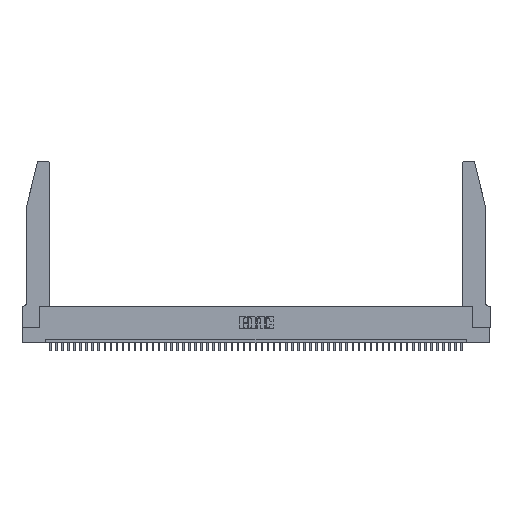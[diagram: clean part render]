
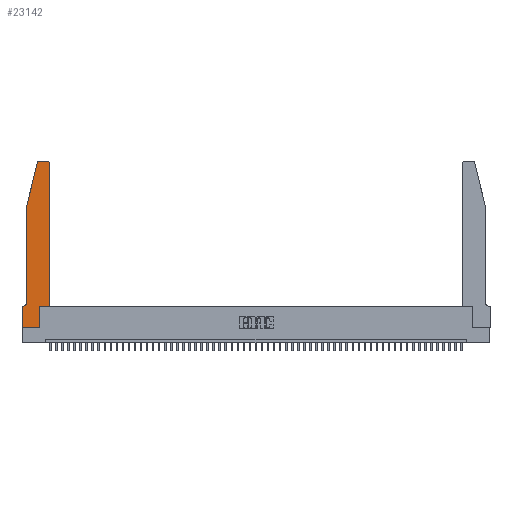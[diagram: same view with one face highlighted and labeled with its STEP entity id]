
A CAD part, top view. The second image highlights one B-rep face of the part: STEP entity #23142.
In plain terms, the highlighted planar face has unit normal (0, 0, 1).
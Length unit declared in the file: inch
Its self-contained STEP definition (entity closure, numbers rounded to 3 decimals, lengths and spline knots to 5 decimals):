
#243 = EDGE_LOOP ( 'NONE', ( #18158, #18048, #43038, #37399, #42658, #34288, #34234, #25172, #28379, #49204, #23514, #32683 ) ) ;
#1354 = LINE ( 'NONE', #51757, #47501 ) ;
#1744 = DIRECTION ( 'NONE',  ( 1., 0., 0. ) ) ;
#2928 = AXIS2_PLACEMENT_3D ( 'NONE', #8371, #4436, #11940 ) ;
#3563 = DIRECTION ( 'NONE',  ( -0.239, -0.971, 0. ) ) ;
#4314 = VERTEX_POINT ( 'NONE', #22705 ) ;
#4436 = DIRECTION ( 'NONE',  ( 0., 0., 1. ) ) ;
#4733 = VERTEX_POINT ( 'NONE', #39611 ) ;
#5491 = CARTESIAN_POINT ( 'NONE',  ( 0.4205, 2.72, 0.37 ) ) ;
#6585 = DIRECTION ( 'NONE',  ( 0., -1., 0. ) ) ;
#7000 = EDGE_CURVE ( 'NONE', #42185, #9568, #35794, .T. ) ;
#7491 = CARTESIAN_POINT ( 'NONE',  ( 0.0755, 2., 0.37 ) ) ;
#8063 = DIRECTION ( 'NONE',  ( 0., -1., 0. ) ) ;
#8371 = CARTESIAN_POINT ( 'NONE',  ( 0.284, 2.72, 0.37 ) ) ;
#9288 = LINE ( 'NONE', #7491, #38144 ) ;
#9568 = VERTEX_POINT ( 'NONE', #14014 ) ;
#9901 = LINE ( 'NONE', #24311, #46450 ) ;
#11267 = VECTOR ( 'NONE', #15106, 39.37008 ) ;
#11940 = DIRECTION ( 'NONE',  ( 1., 0., 0. ) ) ;
#13258 = VERTEX_POINT ( 'NONE', #42919 ) ;
#14014 = CARTESIAN_POINT ( 'NONE',  ( 0., 0.35, 0.37 ) ) ;
#14015 = VERTEX_POINT ( 'NONE', #36875 ) ;
#14400 = EDGE_CURVE ( 'NONE', #44410, #52552, #49768, .T. ) ;
#14858 = AXIS2_PLACEMENT_3D ( 'NONE', #26701, #46902, #34383 ) ;
#15106 = DIRECTION ( 'NONE',  ( -1., 0., 0. ) ) ;
#15272 = VECTOR ( 'NONE', #31487, 39.37008 ) ;
#18048 = ORIENTED_EDGE ( 'NONE', *, *, #46040, .T. ) ;
#18158 = ORIENTED_EDGE ( 'NONE', *, *, #37678, .T. ) ;
#18743 = DIRECTION ( 'NONE',  ( 1., 0., 0. ) ) ;
#19446 = CARTESIAN_POINT ( 'NONE',  ( 0.0755, 0.35, 0.37 ) ) ;
#20597 = CARTESIAN_POINT ( 'NONE',  ( 0.0055, 0.35, 0.37 ) ) ;
#20752 = CIRCLE ( 'NONE', #14858, 0.07 ) ;
#22087 = DIRECTION ( 'NONE',  ( 1., 0., 0. ) ) ;
#22111 = EDGE_CURVE ( 'NONE', #49598, #33706, #38552, .T. ) ;
#22705 = CARTESIAN_POINT ( 'NONE',  ( 0., 0., 0.37 ) ) ;
#23142 = ADVANCED_FACE ( 'NONE', ( #51906 ), #30871, .T. ) ;
#23167 = DIRECTION ( 'NONE',  ( 0., 0., 1. ) ) ;
#23514 = ORIENTED_EDGE ( 'NONE', *, *, #40303, .T. ) ;
#24285 = EDGE_CURVE ( 'NONE', #4314, #13258, #43099, .T. ) ;
#24311 = CARTESIAN_POINT ( 'NONE',  ( 0.2865, 0.35, 0.37 ) ) ;
#25172 = ORIENTED_EDGE ( 'NONE', *, *, #24285, .T. ) ;
#26701 = CARTESIAN_POINT ( 'NONE',  ( 0.0055, 0.42, 0.37 ) ) ;
#27271 = DIRECTION ( 'NONE',  ( 1., 0., 0. ) ) ;
#27760 = CARTESIAN_POINT ( 'NONE',  ( 0.4505, 2.72, 0.37 ) ) ;
#28379 = ORIENTED_EDGE ( 'NONE', *, *, #53070, .T. ) ;
#28793 = LINE ( 'NONE', #34871, #29410 ) ;
#29410 = VECTOR ( 'NONE', #51356, 39.37008 ) ;
#30864 = EDGE_CURVE ( 'NONE', #9568, #4314, #1354, .T. ) ;
#30871 = PLANE ( 'NONE',  #45918 ) ;
#31487 = DIRECTION ( 'NONE',  ( -1., 0., 0. ) ) ;
#32683 = ORIENTED_EDGE ( 'NONE', *, *, #14400, .T. ) ;
#32839 = CARTESIAN_POINT ( 'NONE',  ( 0.0755, 2., 0.37 ) ) ;
#32905 = VECTOR ( 'NONE', #18743, 39.37008 ) ;
#33039 = EDGE_CURVE ( 'NONE', #4733, #42185, #20752, .T. ) ;
#33077 = DIRECTION ( 'NONE',  ( 0., 1., 0. ) ) ;
#33706 = VERTEX_POINT ( 'NONE', #46467 ) ;
#34234 = ORIENTED_EDGE ( 'NONE', *, *, #30864, .T. ) ;
#34288 = ORIENTED_EDGE ( 'NONE', *, *, #7000, .T. ) ;
#34333 = CARTESIAN_POINT ( 'NONE',  ( 0., 0., 0.37 ) ) ;
#34354 = CIRCLE ( 'NONE', #2928, 0.03 ) ;
#34383 = DIRECTION ( 'NONE',  ( -1., 0., 0. ) ) ;
#34656 = CARTESIAN_POINT ( 'NONE',  ( 0.25487, 2.72718, 0.37 ) ) ;
#34871 = CARTESIAN_POINT ( 'NONE',  ( 0.4505, 0.35, 0.37 ) ) ;
#35746 = AXIS2_PLACEMENT_3D ( 'NONE', #5491, #50836, #1744 ) ;
#35794 = LINE ( 'NONE', #19446, #15272 ) ;
#36589 = VECTOR ( 'NONE', #8063, 39.37008 ) ;
#36875 = CARTESIAN_POINT ( 'NONE',  ( 0.284, 2.75, 0.37 ) ) ;
#37399 = ORIENTED_EDGE ( 'NONE', *, *, #39576, .T. ) ;
#37678 = EDGE_CURVE ( 'NONE', #52552, #14015, #42075, .T. ) ;
#37771 = VERTEX_POINT ( 'NONE', #53056 ) ;
#38144 = VECTOR ( 'NONE', #3563, 39.37008 ) ;
#38442 = EDGE_CURVE ( 'NONE', #39146, #37771, #9288, .T. ) ;
#38552 = LINE ( 'NONE', #38573, #42374 ) ;
#38573 = CARTESIAN_POINT ( 'NONE',  ( 0.4505, 0.35, 0.37 ) ) ;
#39146 = VERTEX_POINT ( 'NONE', #34656 ) ;
#39576 = EDGE_CURVE ( 'NONE', #37771, #4733, #49403, .T. ) ;
#39593 = CARTESIAN_POINT ( 'NONE',  ( 0., 0.35, 0.37 ) ) ;
#39611 = CARTESIAN_POINT ( 'NONE',  ( 0.0755, 0.42, 0.37 ) ) ;
#40303 = EDGE_CURVE ( 'NONE', #33706, #44410, #28793, .T. ) ;
#42075 = LINE ( 'NONE', #47883, #11267 ) ;
#42185 = VERTEX_POINT ( 'NONE', #20597 ) ;
#42374 = VECTOR ( 'NONE', #22087, 39.37008 ) ;
#42658 = ORIENTED_EDGE ( 'NONE', *, *, #33039, .T. ) ;
#42919 = CARTESIAN_POINT ( 'NONE',  ( 0.2865, 0., 0.37 ) ) ;
#43038 = ORIENTED_EDGE ( 'NONE', *, *, #38442, .T. ) ;
#43099 = LINE ( 'NONE', #34333, #32905 ) ;
#44410 = VERTEX_POINT ( 'NONE', #27760 ) ;
#45429 = CARTESIAN_POINT ( 'NONE',  ( 0.4205, 2.75, 0.37 ) ) ;
#45918 = AXIS2_PLACEMENT_3D ( 'NONE', #39593, #23167, #27271 ) ;
#46040 = EDGE_CURVE ( 'NONE', #14015, #39146, #34354, .T. ) ;
#46450 = VECTOR ( 'NONE', #33077, 39.37008 ) ;
#46467 = CARTESIAN_POINT ( 'NONE',  ( 0.4505, 0.35, 0.37 ) ) ;
#46562 = CARTESIAN_POINT ( 'NONE',  ( 0.2865, 0.35, 0.37 ) ) ;
#46902 = DIRECTION ( 'NONE',  ( 0., 0., -1. ) ) ;
#47501 = VECTOR ( 'NONE', #6585, 39.37008 ) ;
#47883 = CARTESIAN_POINT ( 'NONE',  ( 0.2605, 2.75, 0.37 ) ) ;
#49204 = ORIENTED_EDGE ( 'NONE', *, *, #22111, .T. ) ;
#49403 = LINE ( 'NONE', #32839, #36589 ) ;
#49598 = VERTEX_POINT ( 'NONE', #46562 ) ;
#49768 = CIRCLE ( 'NONE', #35746, 0.03 ) ;
#50836 = DIRECTION ( 'NONE',  ( 0., 0., 1. ) ) ;
#51356 = DIRECTION ( 'NONE',  ( 0., 1., 0. ) ) ;
#51757 = CARTESIAN_POINT ( 'NONE',  ( 0., 0., 0.37 ) ) ;
#51906 = FACE_OUTER_BOUND ( 'NONE', #243, .T. ) ;
#52552 = VERTEX_POINT ( 'NONE', #45429 ) ;
#53056 = CARTESIAN_POINT ( 'NONE',  ( 0.0755, 2., 0.37 ) ) ;
#53070 = EDGE_CURVE ( 'NONE', #13258, #49598, #9901, .T. ) ;
